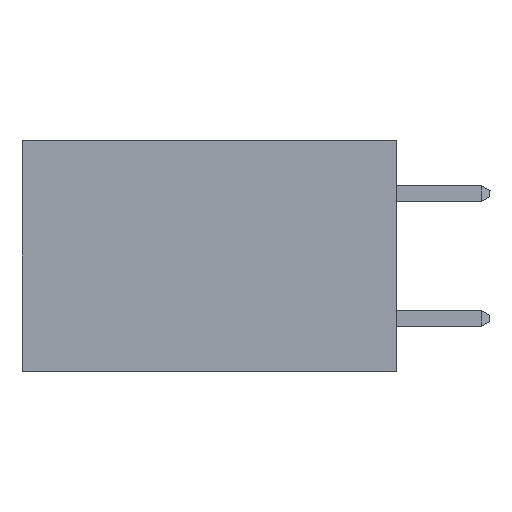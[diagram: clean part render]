
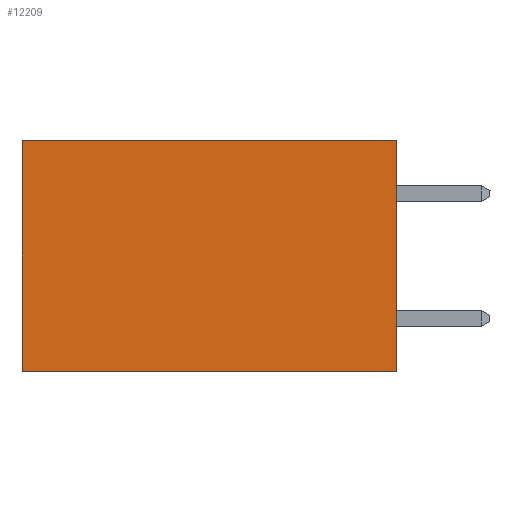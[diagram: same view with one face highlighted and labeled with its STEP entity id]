
A CAD part, left-side view. The second image highlights one B-rep face of the part: STEP entity #12209.
In plain terms, the highlighted planar face has unit normal (-1, 0, 0).
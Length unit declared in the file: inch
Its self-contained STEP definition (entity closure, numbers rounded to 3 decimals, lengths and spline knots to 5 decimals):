
#568 = VECTOR ( 'NONE', #10125, 39.37008 ) ;
#711 = ORIENTED_EDGE ( 'NONE', *, *, #19173, .F. ) ;
#1236 = VECTOR ( 'NONE', #7996, 39.37008 ) ;
#1553 = EDGE_LOOP ( 'NONE', ( #18289, #711, #4356, #5047 ) ) ;
#3248 = EDGE_CURVE ( 'NONE', #7475, #19274, #14846, .T. ) ;
#3801 = CARTESIAN_POINT ( 'NONE',  ( 0.298, 0., -0.37 ) ) ;
#4356 = ORIENTED_EDGE ( 'NONE', *, *, #11904, .F. ) ;
#4754 = CARTESIAN_POINT ( 'NONE',  ( 0.298, 0., 0. ) ) ;
#5047 = ORIENTED_EDGE ( 'NONE', *, *, #3248, .T. ) ;
#5541 = DIRECTION ( 'NONE',  ( 1., 0., 0. ) ) ;
#6495 = CARTESIAN_POINT ( 'NONE',  ( 0.298, 0.6, -0.37 ) ) ;
#6860 = CARTESIAN_POINT ( 'NONE',  ( 0.298, 0., 0. ) ) ;
#6920 = DIRECTION ( 'NONE',  ( 0., 0., -1. ) ) ;
#7115 = CARTESIAN_POINT ( 'NONE',  ( 0.298, 0., 0. ) ) ;
#7475 = VERTEX_POINT ( 'NONE', #6860 ) ;
#7479 = EDGE_CURVE ( 'NONE', #19274, #19194, #18871, .T. ) ;
#7996 = DIRECTION ( 'NONE',  ( 0., 1., 0. ) ) ;
#8734 = DIRECTION ( 'NONE',  ( 0., 0., -1. ) ) ;
#9590 = FACE_OUTER_BOUND ( 'NONE', #1553, .T. ) ;
#10125 = DIRECTION ( 'NONE',  ( 0., 0., -1. ) ) ;
#11699 = VERTEX_POINT ( 'NONE', #3801 ) ;
#11904 = EDGE_CURVE ( 'NONE', #7475, #11699, #16350, .T. ) ;
#12129 = CARTESIAN_POINT ( 'NONE',  ( 0.298, 0., -0.37 ) ) ;
#12209 = ADVANCED_FACE ( 'NONE', ( #9590 ), #13775, .F. ) ;
#12742 = VECTOR ( 'NONE', #15420, 39.37008 ) ;
#13658 = CARTESIAN_POINT ( 'NONE',  ( 0.298, 0.6, 0. ) ) ;
#13775 = PLANE ( 'NONE',  #18333 ) ;
#14846 = LINE ( 'NONE', #4754, #1236 ) ;
#15143 = CARTESIAN_POINT ( 'NONE',  ( 0.298, 0., 0. ) ) ;
#15420 = DIRECTION ( 'NONE',  ( 0., 1., 0. ) ) ;
#15806 = CARTESIAN_POINT ( 'NONE',  ( 0.298, 0.6, 0. ) ) ;
#16350 = LINE ( 'NONE', #15143, #16874 ) ;
#16874 = VECTOR ( 'NONE', #6920, 39.37008 ) ;
#17168 = LINE ( 'NONE', #12129, #12742 ) ;
#18289 = ORIENTED_EDGE ( 'NONE', *, *, #7479, .T. ) ;
#18333 = AXIS2_PLACEMENT_3D ( 'NONE', #7115, #5541, #8734 ) ;
#18871 = LINE ( 'NONE', #13658, #568 ) ;
#19173 = EDGE_CURVE ( 'NONE', #11699, #19194, #17168, .T. ) ;
#19194 = VERTEX_POINT ( 'NONE', #6495 ) ;
#19274 = VERTEX_POINT ( 'NONE', #15806 ) ;
